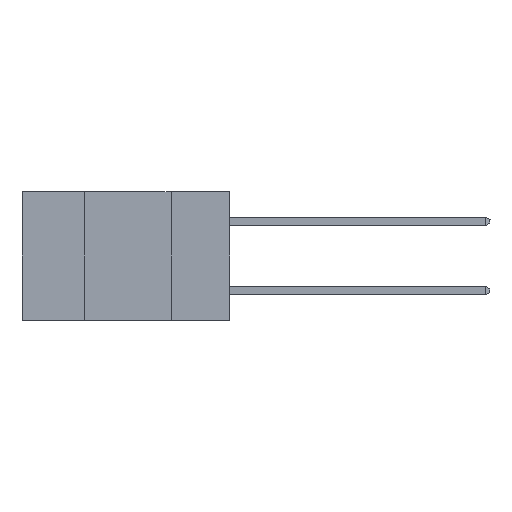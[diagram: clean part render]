
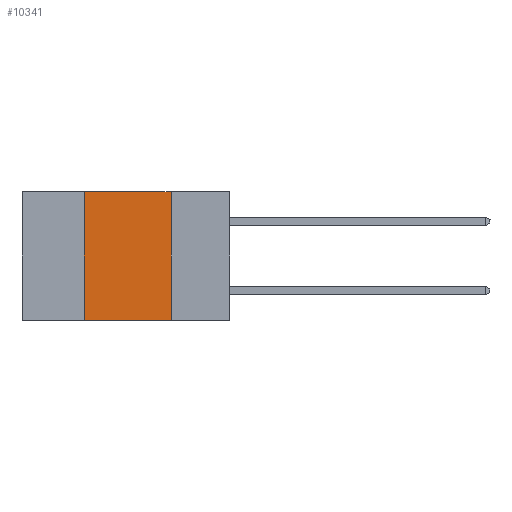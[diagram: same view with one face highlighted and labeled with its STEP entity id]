
A CAD part, left-side view. The second image highlights one B-rep face of the part: STEP entity #10341.
In plain terms, the highlighted planar face has unit normal (-1, 0, 0).
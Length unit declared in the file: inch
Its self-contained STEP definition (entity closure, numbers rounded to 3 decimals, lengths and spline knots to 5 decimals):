
#343 = VERTEX_POINT ( 'NONE', #8600 ) ;
#771 = LINE ( 'NONE', #15163, #5018 ) ;
#1225 = CARTESIAN_POINT ( 'NONE',  ( 0., 0.42, -0.37 ) ) ;
#1722 = EDGE_LOOP ( 'NONE', ( #15143, #11401, #19729, #3431 ) ) ;
#2142 = CARTESIAN_POINT ( 'NONE',  ( 0., 0.42, 0. ) ) ;
#2359 = VECTOR ( 'NONE', #15809, 39.37008 ) ;
#2632 = VERTEX_POINT ( 'NONE', #4071 ) ;
#3431 = ORIENTED_EDGE ( 'NONE', *, *, #13212, .T. ) ;
#3594 = EDGE_CURVE ( 'NONE', #343, #18865, #771, .T. ) ;
#4071 = CARTESIAN_POINT ( 'NONE',  ( 0., 0.42, 0. ) ) ;
#5018 = VECTOR ( 'NONE', #15139, 39.37008 ) ;
#5716 = VECTOR ( 'NONE', #17138, 39.37008 ) ;
#7090 = PLANE ( 'NONE',  #14404 ) ;
#7702 = CARTESIAN_POINT ( 'NONE',  ( 0., 0.6, -0.37 ) ) ;
#7892 = EDGE_CURVE ( 'NONE', #12618, #2632, #12337, .T. ) ;
#8600 = CARTESIAN_POINT ( 'NONE',  ( 0., 0.17, 0. ) ) ;
#8826 = FACE_OUTER_BOUND ( 'NONE', #1722, .T. ) ;
#10246 = EDGE_CURVE ( 'NONE', #2632, #343, #15597, .T. ) ;
#10341 = ADVANCED_FACE ( 'NONE', ( #8826 ), #7090, .F. ) ;
#10351 = DIRECTION ( 'NONE',  ( 0., 0., -1. ) ) ;
#11401 = ORIENTED_EDGE ( 'NONE', *, *, #10246, .F. ) ;
#11695 = DIRECTION ( 'NONE',  ( 0., 0., 1. ) ) ;
#12337 = LINE ( 'NONE', #2142, #16551 ) ;
#12599 = CARTESIAN_POINT ( 'NONE',  ( 0., 0.6, 0. ) ) ;
#12618 = VERTEX_POINT ( 'NONE', #1225 ) ;
#13212 = EDGE_CURVE ( 'NONE', #12618, #18865, #14214, .T. ) ;
#14214 = LINE ( 'NONE', #7702, #5716 ) ;
#14404 = AXIS2_PLACEMENT_3D ( 'NONE', #18236, #19756, #10351 ) ;
#15139 = DIRECTION ( 'NONE',  ( 0., 0., -1. ) ) ;
#15143 = ORIENTED_EDGE ( 'NONE', *, *, #3594, .F. ) ;
#15163 = CARTESIAN_POINT ( 'NONE',  ( 0., 0.17, 0. ) ) ;
#15597 = LINE ( 'NONE', #12599, #2359 ) ;
#15809 = DIRECTION ( 'NONE',  ( 0., -1., 0. ) ) ;
#16551 = VECTOR ( 'NONE', #11695, 39.37008 ) ;
#17138 = DIRECTION ( 'NONE',  ( 0., -1., 0. ) ) ;
#18236 = CARTESIAN_POINT ( 'NONE',  ( 0., 0.6, 0. ) ) ;
#18865 = VERTEX_POINT ( 'NONE', #19323 ) ;
#19323 = CARTESIAN_POINT ( 'NONE',  ( 0., 0.17, -0.37 ) ) ;
#19729 = ORIENTED_EDGE ( 'NONE', *, *, #7892, .F. ) ;
#19756 = DIRECTION ( 'NONE',  ( 1., 0., 0. ) ) ;
